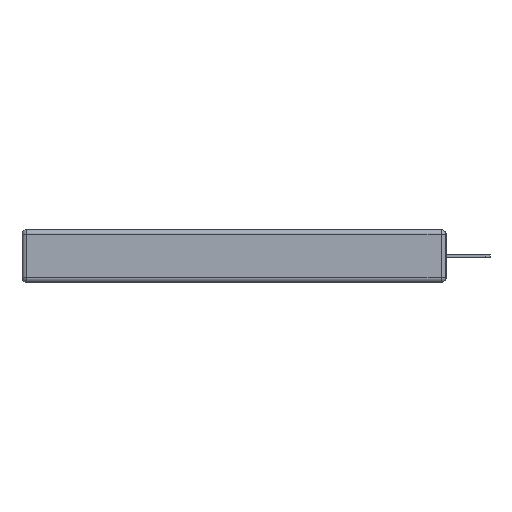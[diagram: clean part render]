
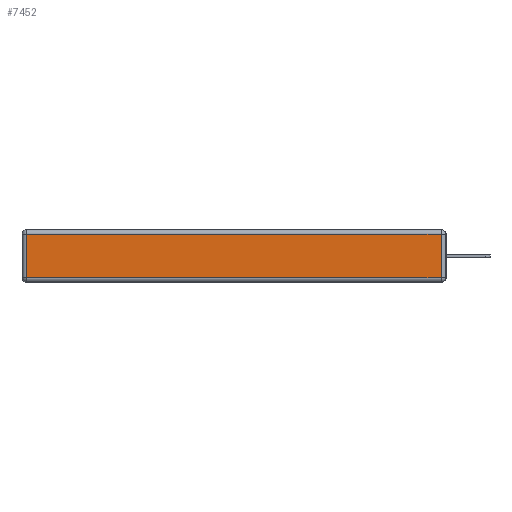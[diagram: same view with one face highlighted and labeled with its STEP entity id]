
A CAD part, left-side view. The second image highlights one B-rep face of the part: STEP entity #7452.
In plain terms, the highlighted planar face has unit normal (-1, 0, 0).
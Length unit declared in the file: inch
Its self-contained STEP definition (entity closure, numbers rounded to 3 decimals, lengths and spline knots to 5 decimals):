
#214 = DIRECTION ( 'NONE',  ( 0., 1., 0. ) ) ;
#735 = ORIENTED_EDGE ( 'NONE', *, *, #6892, .T. ) ;
#1202 = DIRECTION ( 'NONE',  ( 0., 0., 1. ) ) ;
#1844 = LINE ( 'NONE', #9234, #2200 ) ;
#1851 = EDGE_LOOP ( 'NONE', ( #11832, #8809, #9899, #735 ) ) ;
#2053 = CARTESIAN_POINT ( 'NONE',  ( 0., 0.03, -0.03 ) ) ;
#2200 = VECTOR ( 'NONE', #3406, 39.37008 ) ;
#2283 = VECTOR ( 'NONE', #1202, 39.37008 ) ;
#3282 = VERTEX_POINT ( 'NONE', #10848 ) ;
#3406 = DIRECTION ( 'NONE',  ( 0., -1., 0. ) ) ;
#3537 = DIRECTION ( 'NONE',  ( 0., 0., 1. ) ) ;
#3541 = CARTESIAN_POINT ( 'NONE',  ( 0., 0.03, -0.313 ) ) ;
#3756 = EDGE_CURVE ( 'NONE', #9825, #11291, #1844, .T. ) ;
#4738 = PLANE ( 'NONE',  #12380 ) ;
#5284 = LINE ( 'NONE', #9035, #2283 ) ;
#5794 = CARTESIAN_POINT ( 'NONE',  ( 0., 0., -0.343 ) ) ;
#5905 = CARTESIAN_POINT ( 'NONE',  ( 0., 2.75, -0.03 ) ) ;
#6892 = EDGE_CURVE ( 'NONE', #3282, #9825, #11272, .T. ) ;
#6988 = DIRECTION ( 'NONE',  ( -1., 0., 0. ) ) ;
#7452 = ADVANCED_FACE ( 'NONE', ( #8184 ), #4738, .T. ) ;
#8184 = FACE_OUTER_BOUND ( 'NONE', #1851, .T. ) ;
#8793 = CARTESIAN_POINT ( 'NONE',  ( 0., 2.72, -0.313 ) ) ;
#8809 = ORIENTED_EDGE ( 'NONE', *, *, #12168, .T. ) ;
#9035 = CARTESIAN_POINT ( 'NONE',  ( 0., 0.03, -0.343 ) ) ;
#9207 = LINE ( 'NONE', #5905, #9389 ) ;
#9234 = CARTESIAN_POINT ( 'NONE',  ( 0., 0., -0.313 ) ) ;
#9389 = VECTOR ( 'NONE', #214, 39.37008 ) ;
#9452 = VECTOR ( 'NONE', #10875, 39.37008 ) ;
#9808 = CARTESIAN_POINT ( 'NONE',  ( 0., 2.72, -0.343 ) ) ;
#9825 = VERTEX_POINT ( 'NONE', #8793 ) ;
#9899 = ORIENTED_EDGE ( 'NONE', *, *, #14709, .T. ) ;
#10848 = CARTESIAN_POINT ( 'NONE',  ( 0., 2.72, -0.03 ) ) ;
#10875 = DIRECTION ( 'NONE',  ( 0., 0., -1. ) ) ;
#11272 = LINE ( 'NONE', #9808, #9452 ) ;
#11291 = VERTEX_POINT ( 'NONE', #3541 ) ;
#11832 = ORIENTED_EDGE ( 'NONE', *, *, #3756, .T. ) ;
#12168 = EDGE_CURVE ( 'NONE', #11291, #13871, #5284, .T. ) ;
#12380 = AXIS2_PLACEMENT_3D ( 'NONE', #5794, #6988, #3537 ) ;
#13871 = VERTEX_POINT ( 'NONE', #2053 ) ;
#14709 = EDGE_CURVE ( 'NONE', #13871, #3282, #9207, .T. ) ;
